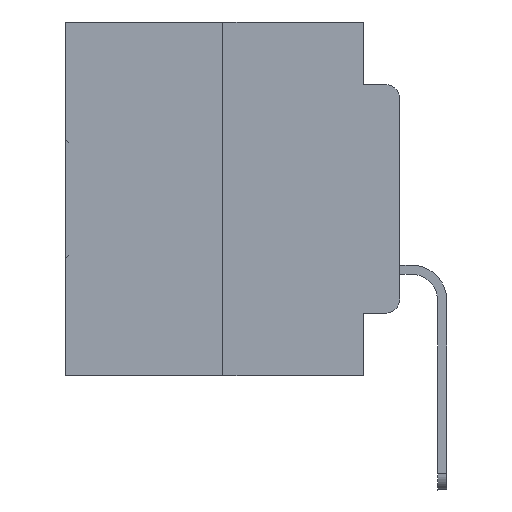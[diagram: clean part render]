
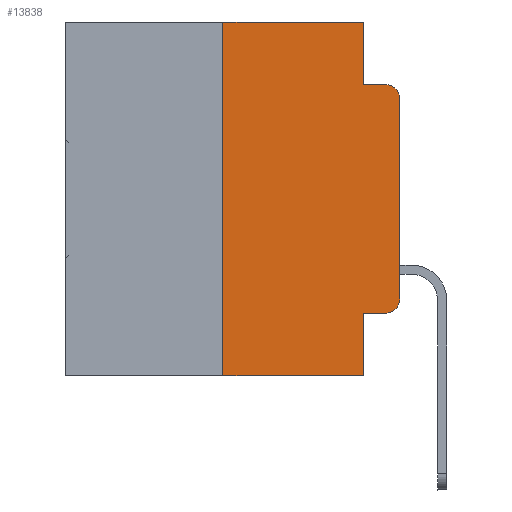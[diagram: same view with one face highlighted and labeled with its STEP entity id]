
A CAD part, left-side view. The second image highlights one B-rep face of the part: STEP entity #13838.
In plain terms, the highlighted planar face has unit normal (-1, 0, 0).
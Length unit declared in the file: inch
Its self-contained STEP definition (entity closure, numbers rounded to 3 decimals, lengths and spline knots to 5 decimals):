
#137 = DIRECTION ( 'NONE',  ( 1., 0., 0. ) ) ;
#634 = EDGE_CURVE ( 'NONE', #20930, #3303, #24694, .T. ) ;
#1133 = EDGE_CURVE ( 'NONE', #12797, #12730, #26419, .T. ) ;
#1144 = VECTOR ( 'NONE', #17835, 39.37008 ) ;
#1698 = CARTESIAN_POINT ( 'NONE',  ( 0., 0.02, -0.1085 ) ) ;
#2131 = CARTESIAN_POINT ( 'NONE',  ( 0., 0.051, 0. ) ) ;
#2429 = CARTESIAN_POINT ( 'NONE',  ( 0., 0.051, 0. ) ) ;
#2479 = CARTESIAN_POINT ( 'NONE',  ( 0., 0., 0. ) ) ;
#2662 = EDGE_LOOP ( 'NONE', ( #13414, #23644, #2745, #14694, #25111, #9922, #17822, #25903, #23539, #25264 ) ) ;
#2745 = ORIENTED_EDGE ( 'NONE', *, *, #634, .F. ) ;
#2942 = CARTESIAN_POINT ( 'NONE',  ( 0., 0., -0.1085 ) ) ;
#3303 = VERTEX_POINT ( 'NONE', #6834 ) ;
#4605 = VECTOR ( 'NONE', #7996, 39.37008 ) ;
#4743 = VERTEX_POINT ( 'NONE', #21974 ) ;
#4965 = DIRECTION ( 'NONE',  ( 0., 0., -1. ) ) ;
#5362 = DIRECTION ( 'NONE',  ( 0., -1., 0. ) ) ;
#5409 = DIRECTION ( 'NONE',  ( 0., -1., 0. ) ) ;
#5991 = DIRECTION ( 'NONE',  ( -1., 0., 0. ) ) ;
#6108 = EDGE_CURVE ( 'NONE', #29837, #3303, #18594, .T. ) ;
#6198 = EDGE_CURVE ( 'NONE', #12730, #29837, #9146, .T. ) ;
#6834 = CARTESIAN_POINT ( 'NONE',  ( 0., 0.02, -0.0885 ) ) ;
#7055 = DIRECTION ( 'NONE',  ( 0., 0., -1. ) ) ;
#7526 = LINE ( 'NONE', #22486, #4605 ) ;
#7736 = LINE ( 'NONE', #27140, #19364 ) ;
#7996 = DIRECTION ( 'NONE',  ( 0., -1., 0. ) ) ;
#9146 = LINE ( 'NONE', #2479, #19969 ) ;
#9444 = CARTESIAN_POINT ( 'NONE',  ( 0., 0.02, -0.3915 ) ) ;
#9497 = VECTOR ( 'NONE', #21903, 39.37008 ) ;
#9739 = LINE ( 'NONE', #2429, #18070 ) ;
#9922 = ORIENTED_EDGE ( 'NONE', *, *, #28887, .F. ) ;
#10329 = CARTESIAN_POINT ( 'NONE',  ( 0., 0.473, 0. ) ) ;
#10486 = LINE ( 'NONE', #10329, #16570 ) ;
#11212 = EDGE_CURVE ( 'NONE', #15020, #12797, #7526, .T. ) ;
#11395 = DIRECTION ( 'NONE',  ( -1., 0., 0. ) ) ;
#12730 = VERTEX_POINT ( 'NONE', #31346 ) ;
#12797 = VERTEX_POINT ( 'NONE', #18963 ) ;
#12911 = CARTESIAN_POINT ( 'NONE',  ( 0., 0.051, 0. ) ) ;
#13414 = ORIENTED_EDGE ( 'NONE', *, *, #6198, .T. ) ;
#13838 = ADVANCED_FACE ( 'NONE', ( #16981 ), #26210, .F. ) ;
#14234 = DIRECTION ( 'NONE',  ( 0., 0., 1. ) ) ;
#14694 = ORIENTED_EDGE ( 'NONE', *, *, #27944, .F. ) ;
#15020 = VERTEX_POINT ( 'NONE', #28181 ) ;
#15158 = CARTESIAN_POINT ( 'NONE',  ( 0., 0.25, -0.5 ) ) ;
#15623 = EDGE_CURVE ( 'NONE', #15948, #4743, #7736, .T. ) ;
#15948 = VERTEX_POINT ( 'NONE', #15158 ) ;
#16570 = VECTOR ( 'NONE', #5409, 39.37008 ) ;
#16848 = CARTESIAN_POINT ( 'NONE',  ( 0., 0.051, -0.0885 ) ) ;
#16981 = FACE_OUTER_BOUND ( 'NONE', #2662, .T. ) ;
#17397 = CARTESIAN_POINT ( 'NONE',  ( 0., 0.25, 0. ) ) ;
#17666 = LINE ( 'NONE', #12911, #28656 ) ;
#17822 = ORIENTED_EDGE ( 'NONE', *, *, #15623, .T. ) ;
#17835 = DIRECTION ( 'NONE',  ( 0., -1., 0. ) ) ;
#18070 = VECTOR ( 'NONE', #4965, 39.37008 ) ;
#18594 = CIRCLE ( 'NONE', #26728, 0.02 ) ;
#18963 = CARTESIAN_POINT ( 'NONE',  ( 0., 0.02, -0.4115 ) ) ;
#19364 = VECTOR ( 'NONE', #5362, 39.37008 ) ;
#19694 = DIRECTION ( 'NONE',  ( 0., 0., -1. ) ) ;
#19969 = VECTOR ( 'NONE', #14234, 39.37008 ) ;
#20679 = EDGE_CURVE ( 'NONE', #15020, #4743, #17666, .T. ) ;
#20843 = AXIS2_PLACEMENT_3D ( 'NONE', #9444, #5991, #7055 ) ;
#20930 = VERTEX_POINT ( 'NONE', #16848 ) ;
#21098 = DIRECTION ( 'NONE',  ( 0., 0., -1. ) ) ;
#21903 = DIRECTION ( 'NONE',  ( 0., 0., 1. ) ) ;
#21974 = CARTESIAN_POINT ( 'NONE',  ( 0., 0.051, -0.5 ) ) ;
#22486 = CARTESIAN_POINT ( 'NONE',  ( 0., 0.051, -0.4115 ) ) ;
#23539 = ORIENTED_EDGE ( 'NONE', *, *, #11212, .T. ) ;
#23644 = ORIENTED_EDGE ( 'NONE', *, *, #6108, .T. ) ;
#24281 = CARTESIAN_POINT ( 'NONE',  ( 0., 0.25, 0. ) ) ;
#24694 = LINE ( 'NONE', #29780, #1144 ) ;
#25111 = ORIENTED_EDGE ( 'NONE', *, *, #28480, .F. ) ;
#25264 = ORIENTED_EDGE ( 'NONE', *, *, #1133, .T. ) ;
#25290 = DIRECTION ( 'NONE',  ( 0., 0., -1. ) ) ;
#25903 = ORIENTED_EDGE ( 'NONE', *, *, #20679, .F. ) ;
#26210 = PLANE ( 'NONE',  #26461 ) ;
#26419 = CIRCLE ( 'NONE', #20843, 0.02 ) ;
#26461 = AXIS2_PLACEMENT_3D ( 'NONE', #26688, #137, #19694 ) ;
#26688 = CARTESIAN_POINT ( 'NONE',  ( 0., 0.473, 0. ) ) ;
#26728 = AXIS2_PLACEMENT_3D ( 'NONE', #1698, #11395, #21098 ) ;
#26816 = LINE ( 'NONE', #24281, #9497 ) ;
#27140 = CARTESIAN_POINT ( 'NONE',  ( 0., 0.473, -0.5 ) ) ;
#27944 = EDGE_CURVE ( 'NONE', #31285, #20930, #9739, .T. ) ;
#28181 = CARTESIAN_POINT ( 'NONE',  ( 0., 0.051, -0.4115 ) ) ;
#28480 = EDGE_CURVE ( 'NONE', #29355, #31285, #10486, .T. ) ;
#28656 = VECTOR ( 'NONE', #25290, 39.37008 ) ;
#28887 = EDGE_CURVE ( 'NONE', #15948, #29355, #26816, .T. ) ;
#29355 = VERTEX_POINT ( 'NONE', #17397 ) ;
#29780 = CARTESIAN_POINT ( 'NONE',  ( 0., 0.051, -0.0885 ) ) ;
#29837 = VERTEX_POINT ( 'NONE', #2942 ) ;
#31285 = VERTEX_POINT ( 'NONE', #2131 ) ;
#31346 = CARTESIAN_POINT ( 'NONE',  ( 0., 0., -0.3915 ) ) ;
